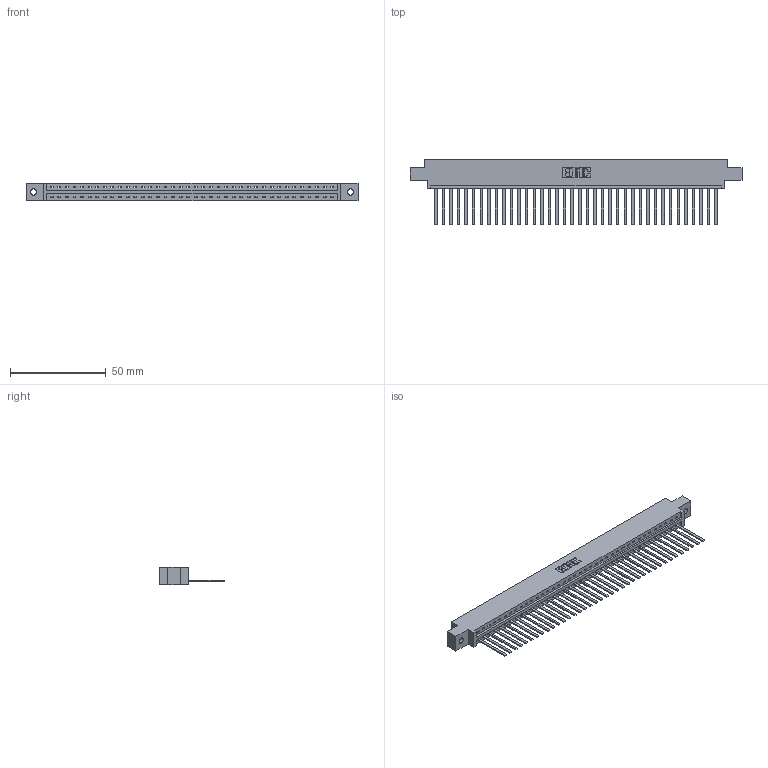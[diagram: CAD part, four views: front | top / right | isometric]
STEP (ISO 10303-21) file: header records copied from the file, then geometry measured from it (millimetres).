
FILE_DESCRIPTION (( 'STEP AP203' ), '1' );
FILE_NAME ('387-038-544-602.STEP', '2018-09-19T05:59:43', ( '' ), ( '' ), 'SwSTEP 2.0', 'SolidWorks 2016', '' );
FILE_SCHEMA (( 'CONFIG_CONTROL_DESIGN' ));
Length unit declared in the file: inch
Products named in the file (3): 337 Part_0.170 Offset - 0.128 Dia; 345-292-001_345-293-144; 387-038-544-602
Assembly tree (39 placements, depth 2):
  387-038-544-602
    337 Part_0.170 Offset - 0.128 Dia
    345-292-001_345-293-144  x38
Bounding box: 173.58 x 34.3 x 9.4 mm (x, y, z)
Volume: 18276.9 mm3; surface area: 20138.6 mm2
Topology: 39 solids, 39 shells, 2246 faces, 6783 edges, 4470 vertices
Faces by surface type: plane 1670, cylinder 576
Entity records: 28715 total; most frequent: CARTESIAN_POINT 5008, ORIENTED_EDGE 4982, DIRECTION 4219, EDGE_CURVE 2491, LINE 2367, VECTOR 2367, VERTEX_POINT 1658, AXIS2_PLACEMENT_3D 926
